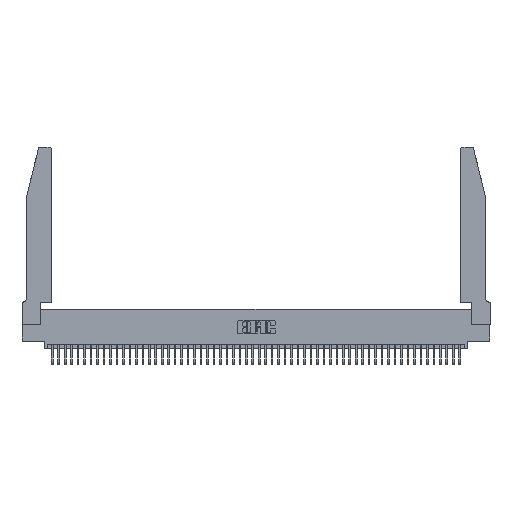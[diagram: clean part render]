
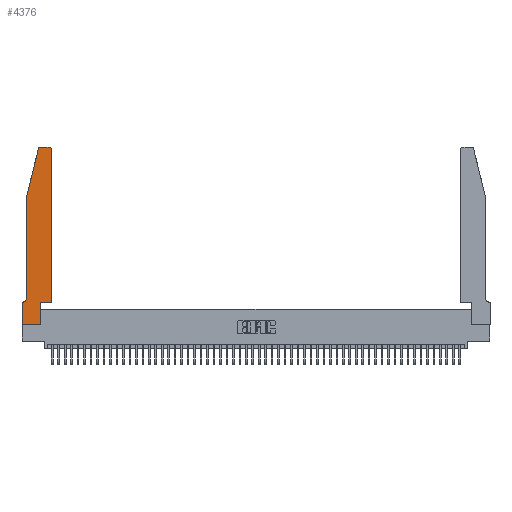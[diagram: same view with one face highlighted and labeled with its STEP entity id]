
A CAD part, top view. The second image highlights one B-rep face of the part: STEP entity #4376.
In plain terms, the highlighted planar face has unit normal (0, 0, 1).
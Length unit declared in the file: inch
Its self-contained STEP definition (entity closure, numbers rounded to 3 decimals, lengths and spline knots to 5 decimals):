
#1338 = CARTESIAN_POINT ( 'NONE',  ( 0., 0.35, 0.37 ) ) ;
#1352 = ORIENTED_EDGE ( 'NONE', *, *, #1428, .T. ) ;
#1428 = EDGE_CURVE ( 'NONE', #45881, #36635, #30755, .T. ) ;
#3362 = EDGE_CURVE ( 'NONE', #31698, #30044, #4552, .T. ) ;
#3440 = DIRECTION ( 'NONE',  ( 1., 0., 0. ) ) ;
#4364 = EDGE_CURVE ( 'NONE', #30089, #16459, #8727, .T. ) ;
#4376 = ADVANCED_FACE ( 'NONE', ( #47416 ), #24721, .T. ) ;
#4552 = CIRCLE ( 'NONE', #34144, 0.03 ) ;
#4707 = LINE ( 'NONE', #6410, #25415 ) ;
#5093 = CIRCLE ( 'NONE', #43620, 0.03 ) ;
#5311 = DIRECTION ( 'NONE',  ( 0., 0., 1. ) ) ;
#5758 = ORIENTED_EDGE ( 'NONE', *, *, #14314, .T. ) ;
#5882 = EDGE_LOOP ( 'NONE', ( #14072, #28597, #22323, #18219, #1352, #30437, #41676, #27189, #7851, #5758, #31937, #49308 ) ) ;
#6410 = CARTESIAN_POINT ( 'NONE',  ( 0.0755, 2., 0.37 ) ) ;
#6694 = VERTEX_POINT ( 'NONE', #15716 ) ;
#7197 = EDGE_CURVE ( 'NONE', #16459, #45881, #4707, .T. ) ;
#7509 = VECTOR ( 'NONE', #40057, 39.37008 ) ;
#7756 = LINE ( 'NONE', #45388, #27185 ) ;
#7851 = ORIENTED_EDGE ( 'NONE', *, *, #25440, .T. ) ;
#7887 = DIRECTION ( 'NONE',  ( 1., 0., 0. ) ) ;
#8591 = EDGE_CURVE ( 'NONE', #6694, #24674, #13770, .T. ) ;
#8727 = LINE ( 'NONE', #31563, #7509 ) ;
#8785 = CARTESIAN_POINT ( 'NONE',  ( 0.284, 2.75, 0.37 ) ) ;
#10150 = VERTEX_POINT ( 'NONE', #24675 ) ;
#10975 = EDGE_CURVE ( 'NONE', #24674, #33458, #46075, .T. ) ;
#11086 = CARTESIAN_POINT ( 'NONE',  ( 0.4505, 2.72, 0.37 ) ) ;
#12254 = CARTESIAN_POINT ( 'NONE',  ( 0.4205, 2.75, 0.37 ) ) ;
#12514 = VECTOR ( 'NONE', #45830, 39.37008 ) ;
#13170 = AXIS2_PLACEMENT_3D ( 'NONE', #1338, #5311, #32412 ) ;
#13404 = DIRECTION ( 'NONE',  ( 0., -1., 0. ) ) ;
#13469 = VECTOR ( 'NONE', #7887, 39.37008 ) ;
#13770 = LINE ( 'NONE', #14998, #12514 ) ;
#13840 = VECTOR ( 'NONE', #38176, 39.37008 ) ;
#14072 = ORIENTED_EDGE ( 'NONE', *, *, #42250, .T. ) ;
#14314 = EDGE_CURVE ( 'NONE', #10150, #17192, #33973, .T. ) ;
#14785 = CARTESIAN_POINT ( 'NONE',  ( 0.2865, 0., 0.37 ) ) ;
#14998 = CARTESIAN_POINT ( 'NONE',  ( 0., 0., 0.37 ) ) ;
#15061 = LINE ( 'NONE', #49723, #13840 ) ;
#15716 = CARTESIAN_POINT ( 'NONE',  ( 0., 0.35, 0.37 ) ) ;
#16459 = VERTEX_POINT ( 'NONE', #27458 ) ;
#17192 = VERTEX_POINT ( 'NONE', #43757 ) ;
#17806 = VECTOR ( 'NONE', #21564, 39.37008 ) ;
#18063 = CARTESIAN_POINT ( 'NONE',  ( 0.0055, 0.42, 0.37 ) ) ;
#18219 = ORIENTED_EDGE ( 'NONE', *, *, #7197, .T. ) ;
#18563 = CARTESIAN_POINT ( 'NONE',  ( 0.0755, 0.42, 0.37 ) ) ;
#18945 = EDGE_CURVE ( 'NONE', #22876, #30089, #5093, .T. ) ;
#21083 = EDGE_CURVE ( 'NONE', #36635, #6694, #15061, .T. ) ;
#21564 = DIRECTION ( 'NONE',  ( 1., 0., 0. ) ) ;
#21691 = CARTESIAN_POINT ( 'NONE',  ( 0.284, 2.72, 0.37 ) ) ;
#21921 = DIRECTION ( 'NONE',  ( -1., 0., 0. ) ) ;
#22058 = CARTESIAN_POINT ( 'NONE',  ( 0.2605, 2.75, 0.37 ) ) ;
#22323 = ORIENTED_EDGE ( 'NONE', *, *, #4364, .T. ) ;
#22559 = CARTESIAN_POINT ( 'NONE',  ( 0.4505, 0.35, 0.37 ) ) ;
#22575 = EDGE_CURVE ( 'NONE', #17192, #31698, #23369, .T. ) ;
#22876 = VERTEX_POINT ( 'NONE', #8785 ) ;
#23369 = LINE ( 'NONE', #26488, #42639 ) ;
#24674 = VERTEX_POINT ( 'NONE', #36885 ) ;
#24675 = CARTESIAN_POINT ( 'NONE',  ( 0.2865, 0.35, 0.37 ) ) ;
#24721 = PLANE ( 'NONE',  #13170 ) ;
#25415 = VECTOR ( 'NONE', #13404, 39.37008 ) ;
#25440 = EDGE_CURVE ( 'NONE', #33458, #10150, #7756, .T. ) ;
#25555 = DIRECTION ( 'NONE',  ( 1., 0., 0. ) ) ;
#26488 = CARTESIAN_POINT ( 'NONE',  ( 0.4505, 0.35, 0.37 ) ) ;
#26784 = DIRECTION ( 'NONE',  ( 0., 0., 1. ) ) ;
#27185 = VECTOR ( 'NONE', #33896, 39.37008 ) ;
#27189 = ORIENTED_EDGE ( 'NONE', *, *, #10975, .T. ) ;
#27458 = CARTESIAN_POINT ( 'NONE',  ( 0.0755, 2., 0.37 ) ) ;
#28597 = ORIENTED_EDGE ( 'NONE', *, *, #18945, .T. ) ;
#29279 = CARTESIAN_POINT ( 'NONE',  ( 0., 0., 0.37 ) ) ;
#29761 = DIRECTION ( 'NONE',  ( -1., 0., 0. ) ) ;
#30044 = VERTEX_POINT ( 'NONE', #12254 ) ;
#30089 = VERTEX_POINT ( 'NONE', #43173 ) ;
#30326 = DIRECTION ( 'NONE',  ( 0., 1., 0. ) ) ;
#30437 = ORIENTED_EDGE ( 'NONE', *, *, #21083, .T. ) ;
#30755 = CIRCLE ( 'NONE', #36678, 0.07 ) ;
#31563 = CARTESIAN_POINT ( 'NONE',  ( 0.0755, 2., 0.37 ) ) ;
#31698 = VERTEX_POINT ( 'NONE', #11086 ) ;
#31937 = ORIENTED_EDGE ( 'NONE', *, *, #22575, .T. ) ;
#32412 = DIRECTION ( 'NONE',  ( 1., 0., 0. ) ) ;
#33458 = VERTEX_POINT ( 'NONE', #14785 ) ;
#33896 = DIRECTION ( 'NONE',  ( 0., 1., 0. ) ) ;
#33973 = LINE ( 'NONE', #22559, #13469 ) ;
#34144 = AXIS2_PLACEMENT_3D ( 'NONE', #49803, #26784, #3440 ) ;
#35652 = VECTOR ( 'NONE', #29761, 39.37008 ) ;
#36635 = VERTEX_POINT ( 'NONE', #39250 ) ;
#36678 = AXIS2_PLACEMENT_3D ( 'NONE', #18063, #44966, #21921 ) ;
#36885 = CARTESIAN_POINT ( 'NONE',  ( 0., 0., 0.37 ) ) ;
#36893 = LINE ( 'NONE', #22058, #35652 ) ;
#38176 = DIRECTION ( 'NONE',  ( -1., 0., 0. ) ) ;
#39250 = CARTESIAN_POINT ( 'NONE',  ( 0.0055, 0.35, 0.37 ) ) ;
#40057 = DIRECTION ( 'NONE',  ( -0.239, -0.971, 0. ) ) ;
#41676 = ORIENTED_EDGE ( 'NONE', *, *, #8591, .T. ) ;
#42250 = EDGE_CURVE ( 'NONE', #30044, #22876, #36893, .T. ) ;
#42639 = VECTOR ( 'NONE', #30326, 39.37008 ) ;
#43173 = CARTESIAN_POINT ( 'NONE',  ( 0.25487, 2.72718, 0.37 ) ) ;
#43620 = AXIS2_PLACEMENT_3D ( 'NONE', #21691, #48596, #25555 ) ;
#43757 = CARTESIAN_POINT ( 'NONE',  ( 0.4505, 0.35, 0.37 ) ) ;
#44966 = DIRECTION ( 'NONE',  ( 0., 0., -1. ) ) ;
#45388 = CARTESIAN_POINT ( 'NONE',  ( 0.2865, 0.35, 0.37 ) ) ;
#45830 = DIRECTION ( 'NONE',  ( 0., -1., 0. ) ) ;
#45881 = VERTEX_POINT ( 'NONE', #18563 ) ;
#46075 = LINE ( 'NONE', #29279, #17806 ) ;
#47416 = FACE_OUTER_BOUND ( 'NONE', #5882, .T. ) ;
#48596 = DIRECTION ( 'NONE',  ( 0., 0., 1. ) ) ;
#49308 = ORIENTED_EDGE ( 'NONE', *, *, #3362, .T. ) ;
#49723 = CARTESIAN_POINT ( 'NONE',  ( 0.0755, 0.35, 0.37 ) ) ;
#49803 = CARTESIAN_POINT ( 'NONE',  ( 0.4205, 2.72, 0.37 ) ) ;
